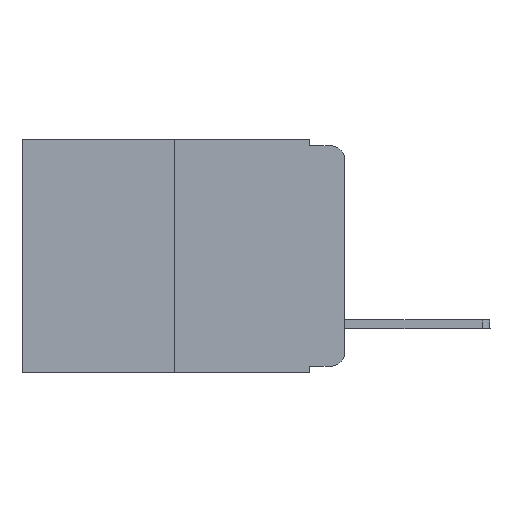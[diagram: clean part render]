
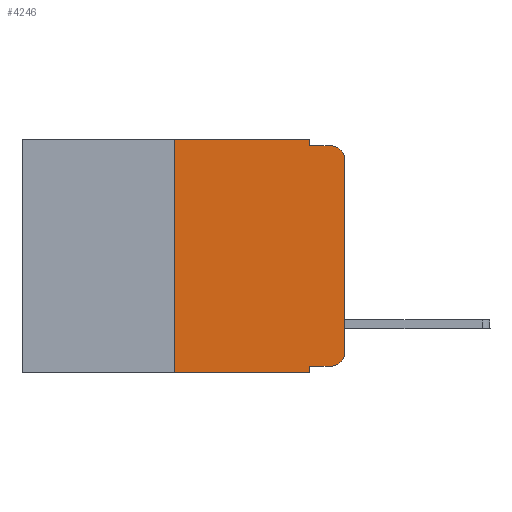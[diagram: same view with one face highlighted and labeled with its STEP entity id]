
A CAD part, left-side view. The second image highlights one B-rep face of the part: STEP entity #4246.
In plain terms, the highlighted planar face has unit normal (-1, 0, 0).
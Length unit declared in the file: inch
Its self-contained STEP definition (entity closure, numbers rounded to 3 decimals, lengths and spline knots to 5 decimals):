
#459 = CARTESIAN_POINT ( 'NONE',  ( 0., 0.02, -0.01 ) ) ;
#608 = VECTOR ( 'NONE', #5163, 39.37008 ) ;
#806 = CIRCLE ( 'NONE', #12675, 0.02 ) ;
#1146 = VECTOR ( 'NONE', #9665, 39.37008 ) ;
#1232 = ORIENTED_EDGE ( 'NONE', *, *, #1980, .F. ) ;
#1355 = CARTESIAN_POINT ( 'NONE',  ( 0., 0.051, -0.343 ) ) ;
#1548 = CARTESIAN_POINT ( 'NONE',  ( 0., 0.02, -0.03 ) ) ;
#1757 = VERTEX_POINT ( 'NONE', #459 ) ;
#1919 = DIRECTION ( 'NONE',  ( 0., 0., 1. ) ) ;
#1975 = ORIENTED_EDGE ( 'NONE', *, *, #4172, .T. ) ;
#1980 = EDGE_CURVE ( 'NONE', #10898, #12277, #12504, .T. ) ;
#2465 = CARTESIAN_POINT ( 'NONE',  ( 0., 0.051, 0. ) ) ;
#3388 = LINE ( 'NONE', #12081, #608 ) ;
#3541 = LINE ( 'NONE', #10708, #11886 ) ;
#3718 = DIRECTION ( 'NONE',  ( 0., -1., 0. ) ) ;
#3835 = EDGE_CURVE ( 'NONE', #4413, #12277, #3388, .T. ) ;
#3956 = CARTESIAN_POINT ( 'NONE',  ( 0., 0., -0.03 ) ) ;
#4106 = LINE ( 'NONE', #13064, #1146 ) ;
#4172 = EDGE_CURVE ( 'NONE', #5951, #9825, #10832, .T. ) ;
#4246 = ADVANCED_FACE ( 'NONE', ( #10470 ), #14915, .F. ) ;
#4413 = VERTEX_POINT ( 'NONE', #13384 ) ;
#4524 = DIRECTION ( 'NONE',  ( 1., 0., 0. ) ) ;
#4750 = DIRECTION ( 'NONE',  ( 0., 0., -1. ) ) ;
#4940 = DIRECTION ( 'NONE',  ( 0., -1., 0. ) ) ;
#5163 = DIRECTION ( 'NONE',  ( 0., -1., 0. ) ) ;
#5165 = ORIENTED_EDGE ( 'NONE', *, *, #7885, .F. ) ;
#5321 = ORIENTED_EDGE ( 'NONE', *, *, #3835, .T. ) ;
#5951 = VERTEX_POINT ( 'NONE', #7702 ) ;
#6015 = ORIENTED_EDGE ( 'NONE', *, *, #11036, .T. ) ;
#6795 = CARTESIAN_POINT ( 'NONE',  ( 0., 0., 0. ) ) ;
#6893 = CARTESIAN_POINT ( 'NONE',  ( 0., 0.02, -0.313 ) ) ;
#6902 = DIRECTION ( 'NONE',  ( 0., 0., -1. ) ) ;
#7095 = AXIS2_PLACEMENT_3D ( 'NONE', #10311, #4524, #14963 ) ;
#7171 = CARTESIAN_POINT ( 'NONE',  ( 0., 0.473, 0. ) ) ;
#7439 = CARTESIAN_POINT ( 'NONE',  ( 0., 0., -0.313 ) ) ;
#7702 = CARTESIAN_POINT ( 'NONE',  ( 0., 0.02, -0.333 ) ) ;
#7712 = VECTOR ( 'NONE', #4750, 39.37008 ) ;
#7885 = EDGE_CURVE ( 'NONE', #4413, #8075, #13954, .T. ) ;
#8037 = VECTOR ( 'NONE', #13791, 39.37008 ) ;
#8075 = VERTEX_POINT ( 'NONE', #11353 ) ;
#8584 = DIRECTION ( 'NONE',  ( 0., 0., -1. ) ) ;
#9061 = DIRECTION ( 'NONE',  ( -1., 0., 0. ) ) ;
#9384 = EDGE_LOOP ( 'NONE', ( #14557, #6015, #9667, #9979, #11116, #5165, #5321, #1232, #11795, #1975 ) ) ;
#9665 = DIRECTION ( 'NONE',  ( 0., -1., 0. ) ) ;
#9667 = ORIENTED_EDGE ( 'NONE', *, *, #12488, .F. ) ;
#9796 = VECTOR ( 'NONE', #3718, 39.37008 ) ;
#9812 = VERTEX_POINT ( 'NONE', #3956 ) ;
#9825 = VERTEX_POINT ( 'NONE', #7439 ) ;
#9830 = VECTOR ( 'NONE', #6902, 39.37008 ) ;
#9979 = ORIENTED_EDGE ( 'NONE', *, *, #12446, .F. ) ;
#9995 = CARTESIAN_POINT ( 'NONE',  ( 0., 0.25, 0. ) ) ;
#10142 = LINE ( 'NONE', #7171, #9796 ) ;
#10311 = CARTESIAN_POINT ( 'NONE',  ( 0., 0.473, 0. ) ) ;
#10470 = FACE_OUTER_BOUND ( 'NONE', #9384, .T. ) ;
#10477 = EDGE_CURVE ( 'NONE', #10898, #5951, #4106, .T. ) ;
#10708 = CARTESIAN_POINT ( 'NONE',  ( 0., 0.051, -0.01 ) ) ;
#10761 = LINE ( 'NONE', #6795, #8037 ) ;
#10806 = LINE ( 'NONE', #2465, #7712 ) ;
#10832 = CIRCLE ( 'NONE', #13596, 0.02 ) ;
#10898 = VERTEX_POINT ( 'NONE', #12530 ) ;
#11022 = EDGE_CURVE ( 'NONE', #8075, #14091, #10142, .T. ) ;
#11036 = EDGE_CURVE ( 'NONE', #9812, #1757, #806, .T. ) ;
#11116 = ORIENTED_EDGE ( 'NONE', *, *, #11022, .F. ) ;
#11323 = CARTESIAN_POINT ( 'NONE',  ( 0., 0.051, 0. ) ) ;
#11353 = CARTESIAN_POINT ( 'NONE',  ( 0., 0.25, 0. ) ) ;
#11795 = ORIENTED_EDGE ( 'NONE', *, *, #10477, .T. ) ;
#11886 = VECTOR ( 'NONE', #4940, 39.37008 ) ;
#12071 = DIRECTION ( 'NONE',  ( -1., 0., 0. ) ) ;
#12081 = CARTESIAN_POINT ( 'NONE',  ( 0., 0.473, -0.343 ) ) ;
#12277 = VERTEX_POINT ( 'NONE', #1355 ) ;
#12446 = EDGE_CURVE ( 'NONE', #14091, #14221, #10806, .T. ) ;
#12488 = EDGE_CURVE ( 'NONE', #14221, #1757, #3541, .T. ) ;
#12504 = LINE ( 'NONE', #13753, #9830 ) ;
#12530 = CARTESIAN_POINT ( 'NONE',  ( 0., 0.051, -0.333 ) ) ;
#12675 = AXIS2_PLACEMENT_3D ( 'NONE', #1548, #12071, #8584 ) ;
#13064 = CARTESIAN_POINT ( 'NONE',  ( 0., 0.051, -0.333 ) ) ;
#13207 = VECTOR ( 'NONE', #1919, 39.37008 ) ;
#13384 = CARTESIAN_POINT ( 'NONE',  ( 0., 0.25, -0.343 ) ) ;
#13596 = AXIS2_PLACEMENT_3D ( 'NONE', #6893, #9061, #15019 ) ;
#13659 = CARTESIAN_POINT ( 'NONE',  ( 0., 0.051, -0.01 ) ) ;
#13753 = CARTESIAN_POINT ( 'NONE',  ( 0., 0.051, 0. ) ) ;
#13759 = EDGE_CURVE ( 'NONE', #9825, #9812, #10761, .T. ) ;
#13791 = DIRECTION ( 'NONE',  ( 0., 0., 1. ) ) ;
#13954 = LINE ( 'NONE', #9995, #13207 ) ;
#14091 = VERTEX_POINT ( 'NONE', #11323 ) ;
#14221 = VERTEX_POINT ( 'NONE', #13659 ) ;
#14557 = ORIENTED_EDGE ( 'NONE', *, *, #13759, .T. ) ;
#14915 = PLANE ( 'NONE',  #7095 ) ;
#14963 = DIRECTION ( 'NONE',  ( 0., 0., -1. ) ) ;
#15019 = DIRECTION ( 'NONE',  ( 0., 0., -1. ) ) ;
